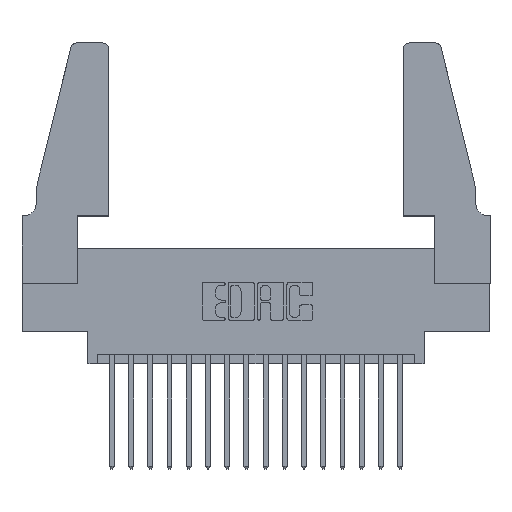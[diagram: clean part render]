
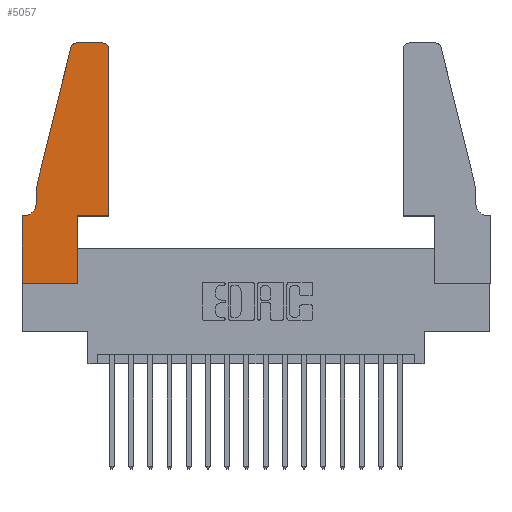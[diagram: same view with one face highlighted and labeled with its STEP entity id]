
A CAD part, top view. The second image highlights one B-rep face of the part: STEP entity #5057.
In plain terms, the highlighted planar face has unit normal (0, 0, 1).
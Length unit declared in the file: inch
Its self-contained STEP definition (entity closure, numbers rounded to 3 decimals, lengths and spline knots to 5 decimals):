
#96 = VECTOR ( 'NONE', #14795, 39.37008 ) ;
#97 = CIRCLE ( 'NONE', #11295, 0.03 ) ;
#160 = CARTESIAN_POINT ( 'NONE',  ( 0.0755, 0.5, 0.37 ) ) ;
#337 = DIRECTION ( 'NONE',  ( -0.239, -0.971, 0. ) ) ;
#792 = CIRCLE ( 'NONE', #17591, 0.03 ) ;
#1243 = EDGE_CURVE ( 'NONE', #2024, #18036, #3256, .T. ) ;
#1273 = CARTESIAN_POINT ( 'NONE',  ( 0.25487, 1.22718, 0.37 ) ) ;
#1414 = EDGE_CURVE ( 'NONE', #18036, #6049, #792, .T. ) ;
#1497 = VECTOR ( 'NONE', #18318, 39.37008 ) ;
#1641 = ORIENTED_EDGE ( 'NONE', *, *, #12058, .T. ) ;
#1730 = CARTESIAN_POINT ( 'NONE',  ( 0.0755, 0.35, 0.37 ) ) ;
#2024 = VERTEX_POINT ( 'NONE', #9113 ) ;
#2058 = VECTOR ( 'NONE', #17467, 39.37008 ) ;
#2256 = ORIENTED_EDGE ( 'NONE', *, *, #2531, .T. ) ;
#2400 = CIRCLE ( 'NONE', #10628, 0.07 ) ;
#2531 = EDGE_CURVE ( 'NONE', #3778, #2024, #5536, .T. ) ;
#2581 = EDGE_CURVE ( 'NONE', #15665, #5921, #8813, .T. ) ;
#2708 = LINE ( 'NONE', #1730, #9446 ) ;
#2905 = FACE_OUTER_BOUND ( 'NONE', #15348, .T. ) ;
#3143 = DIRECTION ( 'NONE',  ( 0., 0., 1. ) ) ;
#3240 = DIRECTION ( 'NONE',  ( 1., 0., 0. ) ) ;
#3256 = LINE ( 'NONE', #5288, #17614 ) ;
#3372 = CARTESIAN_POINT ( 'NONE',  ( 0.4205, 1.22, 0.37 ) ) ;
#3470 = DIRECTION ( 'NONE',  ( 0., 0., 1. ) ) ;
#3576 = DIRECTION ( 'NONE',  ( 0., 0., -1. ) ) ;
#3778 = VERTEX_POINT ( 'NONE', #15641 ) ;
#3965 = PLANE ( 'NONE',  #14129 ) ;
#4146 = LINE ( 'NONE', #13631, #11634 ) ;
#4440 = ORIENTED_EDGE ( 'NONE', *, *, #5929, .T. ) ;
#4513 = EDGE_CURVE ( 'NONE', #5921, #9906, #14559, .T. ) ;
#4834 = ORIENTED_EDGE ( 'NONE', *, *, #2581, .T. ) ;
#4850 = DIRECTION ( 'NONE',  ( 0., 1., 0. ) ) ;
#4917 = CARTESIAN_POINT ( 'NONE',  ( 0.0755, 0.5, 0.37 ) ) ;
#5057 = ADVANCED_FACE ( 'NONE', ( #2905 ), #3965, .T. ) ;
#5252 = ORIENTED_EDGE ( 'NONE', *, *, #1243, .T. ) ;
#5288 = CARTESIAN_POINT ( 'NONE',  ( 0.4505, 0.35, 0.37 ) ) ;
#5536 = LINE ( 'NONE', #17353, #1497 ) ;
#5640 = ORIENTED_EDGE ( 'NONE', *, *, #4513, .T. ) ;
#5921 = VERTEX_POINT ( 'NONE', #4917 ) ;
#5929 = EDGE_CURVE ( 'NONE', #14842, #15665, #97, .T. ) ;
#6049 = VERTEX_POINT ( 'NONE', #7979 ) ;
#6195 = VERTEX_POINT ( 'NONE', #6994 ) ;
#6873 = ORIENTED_EDGE ( 'NONE', *, *, #9688, .T. ) ;
#6909 = LINE ( 'NONE', #16118, #2058 ) ;
#6994 = CARTESIAN_POINT ( 'NONE',  ( 0., 0.35, 0.37 ) ) ;
#7322 = ORIENTED_EDGE ( 'NONE', *, *, #16847, .T. ) ;
#7546 = CARTESIAN_POINT ( 'NONE',  ( 0.0055, 0.35, 0.37 ) ) ;
#7775 = ORIENTED_EDGE ( 'NONE', *, *, #14639, .T. ) ;
#7979 = CARTESIAN_POINT ( 'NONE',  ( 0.4205, 1.25, 0.37 ) ) ;
#8310 = DIRECTION ( 'NONE',  ( 1., 0., 0. ) ) ;
#8428 = EDGE_CURVE ( 'NONE', #12322, #12695, #4146, .T. ) ;
#8813 = LINE ( 'NONE', #160, #15657 ) ;
#8941 = DIRECTION ( 'NONE',  ( -1., 0., 0. ) ) ;
#9034 = ORIENTED_EDGE ( 'NONE', *, *, #1414, .T. ) ;
#9113 = CARTESIAN_POINT ( 'NONE',  ( 0.4505, 0.35, 0.37 ) ) ;
#9446 = VECTOR ( 'NONE', #10433, 39.37008 ) ;
#9524 = DIRECTION ( 'NONE',  ( 1., 0., 0. ) ) ;
#9688 = EDGE_CURVE ( 'NONE', #9906, #16857, #2400, .T. ) ;
#9742 = ORIENTED_EDGE ( 'NONE', *, *, #10384, .T. ) ;
#9906 = VERTEX_POINT ( 'NONE', #17863 ) ;
#10384 = EDGE_CURVE ( 'NONE', #6195, #12322, #15776, .T. ) ;
#10433 = DIRECTION ( 'NONE',  ( -1., 0., 0. ) ) ;
#10628 = AXIS2_PLACEMENT_3D ( 'NONE', #12042, #3576, #13410 ) ;
#10681 = CARTESIAN_POINT ( 'NONE',  ( 0., 0., 0.37 ) ) ;
#10955 = VECTOR ( 'NONE', #16801, 39.37008 ) ;
#11295 = AXIS2_PLACEMENT_3D ( 'NONE', #11931, #3470, #13301 ) ;
#11634 = VECTOR ( 'NONE', #9524, 39.37008 ) ;
#11931 = CARTESIAN_POINT ( 'NONE',  ( 0.284, 1.22, 0.37 ) ) ;
#12042 = CARTESIAN_POINT ( 'NONE',  ( 0.0055, 0.42, 0.37 ) ) ;
#12058 = EDGE_CURVE ( 'NONE', #12695, #3778, #6909, .T. ) ;
#12176 = VECTOR ( 'NONE', #8941, 39.37008 ) ;
#12322 = VERTEX_POINT ( 'NONE', #12627 ) ;
#12627 = CARTESIAN_POINT ( 'NONE',  ( 0., 0., 0.37 ) ) ;
#12695 = VERTEX_POINT ( 'NONE', #15035 ) ;
#13301 = DIRECTION ( 'NONE',  ( 1., 0., 0. ) ) ;
#13410 = DIRECTION ( 'NONE',  ( -1., 0., 0. ) ) ;
#13631 = CARTESIAN_POINT ( 'NONE',  ( 0., 0., 0.37 ) ) ;
#14101 = CARTESIAN_POINT ( 'NONE',  ( 0.0755, 0.5, 0.37 ) ) ;
#14129 = AXIS2_PLACEMENT_3D ( 'NONE', #15143, #16510, #8310 ) ;
#14559 = LINE ( 'NONE', #14101, #10955 ) ;
#14639 = EDGE_CURVE ( 'NONE', #16857, #6195, #2708, .T. ) ;
#14795 = DIRECTION ( 'NONE',  ( 0., -1., 0. ) ) ;
#14842 = VERTEX_POINT ( 'NONE', #17620 ) ;
#15035 = CARTESIAN_POINT ( 'NONE',  ( 0.2865, 0., 0.37 ) ) ;
#15143 = CARTESIAN_POINT ( 'NONE',  ( 0., 0.35, 0.37 ) ) ;
#15309 = ORIENTED_EDGE ( 'NONE', *, *, #8428, .T. ) ;
#15343 = LINE ( 'NONE', #17106, #12176 ) ;
#15348 = EDGE_LOOP ( 'NONE', ( #7322, #4440, #4834, #5640, #6873, #7775, #9742, #15309, #1641, #2256, #5252, #9034 ) ) ;
#15641 = CARTESIAN_POINT ( 'NONE',  ( 0.2865, 0.35, 0.37 ) ) ;
#15657 = VECTOR ( 'NONE', #337, 39.37008 ) ;
#15665 = VERTEX_POINT ( 'NONE', #1273 ) ;
#15776 = LINE ( 'NONE', #10681, #96 ) ;
#15836 = CARTESIAN_POINT ( 'NONE',  ( 0.4505, 1.22, 0.37 ) ) ;
#16118 = CARTESIAN_POINT ( 'NONE',  ( 0.2865, 0.35, 0.37 ) ) ;
#16510 = DIRECTION ( 'NONE',  ( 0., 0., 1. ) ) ;
#16801 = DIRECTION ( 'NONE',  ( 0., -1., 0. ) ) ;
#16847 = EDGE_CURVE ( 'NONE', #6049, #14842, #15343, .T. ) ;
#16857 = VERTEX_POINT ( 'NONE', #7546 ) ;
#17106 = CARTESIAN_POINT ( 'NONE',  ( 0.2605, 1.25, 0.37 ) ) ;
#17353 = CARTESIAN_POINT ( 'NONE',  ( 0.4505, 0.35, 0.37 ) ) ;
#17467 = DIRECTION ( 'NONE',  ( 0., 1., 0. ) ) ;
#17591 = AXIS2_PLACEMENT_3D ( 'NONE', #3372, #3143, #3240 ) ;
#17614 = VECTOR ( 'NONE', #4850, 39.37008 ) ;
#17620 = CARTESIAN_POINT ( 'NONE',  ( 0.284, 1.25, 0.37 ) ) ;
#17863 = CARTESIAN_POINT ( 'NONE',  ( 0.0755, 0.42, 0.37 ) ) ;
#18036 = VERTEX_POINT ( 'NONE', #15836 ) ;
#18318 = DIRECTION ( 'NONE',  ( 1., 0., 0. ) ) ;
